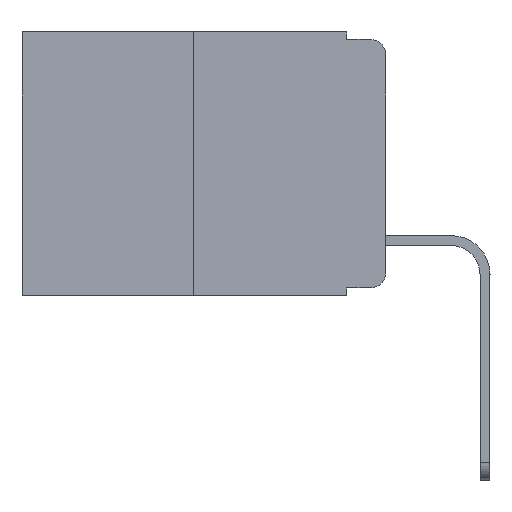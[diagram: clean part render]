
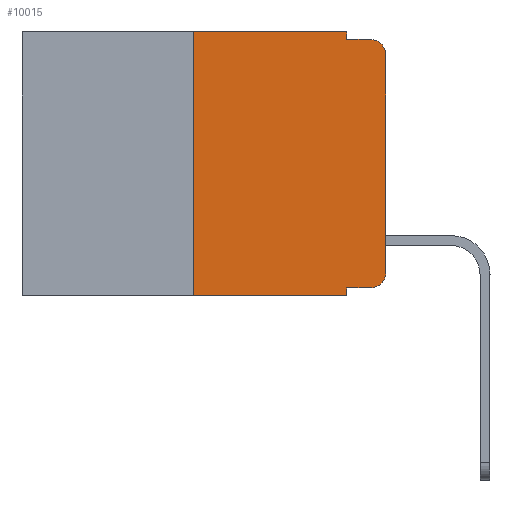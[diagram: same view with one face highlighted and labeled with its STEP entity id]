
A CAD part, left-side view. The second image highlights one B-rep face of the part: STEP entity #10015.
In plain terms, the highlighted planar face has unit normal (-1, 0, 0).
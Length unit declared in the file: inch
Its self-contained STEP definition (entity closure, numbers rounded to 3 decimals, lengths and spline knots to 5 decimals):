
#154 = CARTESIAN_POINT ( 'NONE',  ( 0., 0.051, -0.01 ) ) ;
#623 = ORIENTED_EDGE ( 'NONE', *, *, #19578, .F. ) ;
#699 = CARTESIAN_POINT ( 'NONE',  ( 0., 0.051, 0. ) ) ;
#938 = CARTESIAN_POINT ( 'NONE',  ( 0., 0.051, 0. ) ) ;
#1042 = DIRECTION ( 'NONE',  ( 0., 0., -1. ) ) ;
#1642 = EDGE_CURVE ( 'NONE', #15159, #14908, #9338, .T. ) ;
#1832 = VECTOR ( 'NONE', #19175, 39.37008 ) ;
#2206 = CARTESIAN_POINT ( 'NONE',  ( 0., 0.25, -0.343 ) ) ;
#2340 = ORIENTED_EDGE ( 'NONE', *, *, #16149, .F. ) ;
#3423 = VERTEX_POINT ( 'NONE', #938 ) ;
#4428 = LINE ( 'NONE', #9954, #6712 ) ;
#4862 = CARTESIAN_POINT ( 'NONE',  ( 0., 0., 0. ) ) ;
#5155 = AXIS2_PLACEMENT_3D ( 'NONE', #22812, #6828, #1042 ) ;
#5361 = VERTEX_POINT ( 'NONE', #21335 ) ;
#5397 = DIRECTION ( 'NONE',  ( -1., 0., 0. ) ) ;
#5840 = DIRECTION ( 'NONE',  ( 0., -1., 0. ) ) ;
#5917 = CARTESIAN_POINT ( 'NONE',  ( 0., 0.473, -0.343 ) ) ;
#6068 = DIRECTION ( 'NONE',  ( 0., -1., 0. ) ) ;
#6484 = ORIENTED_EDGE ( 'NONE', *, *, #8996, .T. ) ;
#6598 = DIRECTION ( 'NONE',  ( 0., 0., 1. ) ) ;
#6642 = VERTEX_POINT ( 'NONE', #8885 ) ;
#6712 = VECTOR ( 'NONE', #15363, 39.37008 ) ;
#6759 = DIRECTION ( 'NONE',  ( 0., 0., -1. ) ) ;
#6828 = DIRECTION ( 'NONE',  ( 1., 0., 0. ) ) ;
#6889 = ORIENTED_EDGE ( 'NONE', *, *, #14676, .F. ) ;
#6908 = DIRECTION ( 'NONE',  ( 0., 0., 1. ) ) ;
#7528 = LINE ( 'NONE', #17370, #1832 ) ;
#8420 = EDGE_LOOP ( 'NONE', ( #10664, #22888, #6889, #17474, #623, #2340, #9240, #12591, #6484, #17768 ) ) ;
#8558 = DIRECTION ( 'NONE',  ( 0., -1., 0. ) ) ;
#8692 = EDGE_CURVE ( 'NONE', #20101, #14908, #9041, .T. ) ;
#8847 = AXIS2_PLACEMENT_3D ( 'NONE', #14460, #5397, #14536 ) ;
#8885 = CARTESIAN_POINT ( 'NONE',  ( 0., 0., -0.313 ) ) ;
#8996 = EDGE_CURVE ( 'NONE', #20101, #19986, #18579, .T. ) ;
#9041 = LINE ( 'NONE', #699, #17463 ) ;
#9240 = ORIENTED_EDGE ( 'NONE', *, *, #1642, .T. ) ;
#9338 = LINE ( 'NONE', #5917, #22549 ) ;
#9572 = LINE ( 'NONE', #12081, #19370 ) ;
#9954 = CARTESIAN_POINT ( 'NONE',  ( 0., 0.051, 0. ) ) ;
#10015 = ADVANCED_FACE ( 'NONE', ( #12561 ), #15786, .F. ) ;
#10626 = CIRCLE ( 'NONE', #14514, 0.02 ) ;
#10664 = ORIENTED_EDGE ( 'NONE', *, *, #19601, .T. ) ;
#11359 = VERTEX_POINT ( 'NONE', #17925 ) ;
#11551 = CARTESIAN_POINT ( 'NONE',  ( 0., 0.02, -0.333 ) ) ;
#12081 = CARTESIAN_POINT ( 'NONE',  ( 0., 0.051, -0.01 ) ) ;
#12561 = FACE_OUTER_BOUND ( 'NONE', #8420, .T. ) ;
#12591 = ORIENTED_EDGE ( 'NONE', *, *, #8692, .F. ) ;
#13172 = DIRECTION ( 'NONE',  ( 0., 0., -1. ) ) ;
#14460 = CARTESIAN_POINT ( 'NONE',  ( 0., 0.02, -0.03 ) ) ;
#14514 = AXIS2_PLACEMENT_3D ( 'NONE', #17535, #22961, #6759 ) ;
#14536 = DIRECTION ( 'NONE',  ( 0., 0., -1. ) ) ;
#14676 = EDGE_CURVE ( 'NONE', #20392, #11359, #9572, .T. ) ;
#14908 = VERTEX_POINT ( 'NONE', #23185 ) ;
#15159 = VERTEX_POINT ( 'NONE', #2206 ) ;
#15363 = DIRECTION ( 'NONE',  ( 0., 0., -1. ) ) ;
#15467 = CARTESIAN_POINT ( 'NONE',  ( 0., 0.051, -0.333 ) ) ;
#15786 = PLANE ( 'NONE',  #5155 ) ;
#16149 = EDGE_CURVE ( 'NONE', #15159, #19144, #21340, .T. ) ;
#17370 = CARTESIAN_POINT ( 'NONE',  ( 0., 0.473, 0. ) ) ;
#17447 = VECTOR ( 'NONE', #5840, 39.37008 ) ;
#17463 = VECTOR ( 'NONE', #13172, 39.37008 ) ;
#17474 = ORIENTED_EDGE ( 'NONE', *, *, #18771, .F. ) ;
#17535 = CARTESIAN_POINT ( 'NONE',  ( 0., 0.02, -0.313 ) ) ;
#17768 = ORIENTED_EDGE ( 'NONE', *, *, #19514, .T. ) ;
#17925 = CARTESIAN_POINT ( 'NONE',  ( 0., 0.02, -0.01 ) ) ;
#18579 = LINE ( 'NONE', #20286, #17447 ) ;
#18771 = EDGE_CURVE ( 'NONE', #3423, #20392, #4428, .T. ) ;
#19144 = VERTEX_POINT ( 'NONE', #21785 ) ;
#19175 = DIRECTION ( 'NONE',  ( 0., -1., 0. ) ) ;
#19370 = VECTOR ( 'NONE', #8558, 39.37008 ) ;
#19485 = CIRCLE ( 'NONE', #8847, 0.02 ) ;
#19514 = EDGE_CURVE ( 'NONE', #19986, #6642, #10626, .T. ) ;
#19578 = EDGE_CURVE ( 'NONE', #19144, #3423, #7528, .T. ) ;
#19601 = EDGE_CURVE ( 'NONE', #6642, #5361, #19869, .T. ) ;
#19869 = LINE ( 'NONE', #4862, #21877 ) ;
#19986 = VERTEX_POINT ( 'NONE', #11551 ) ;
#20101 = VERTEX_POINT ( 'NONE', #15467 ) ;
#20286 = CARTESIAN_POINT ( 'NONE',  ( 0., 0.051, -0.333 ) ) ;
#20392 = VERTEX_POINT ( 'NONE', #154 ) ;
#20486 = VECTOR ( 'NONE', #6598, 39.37008 ) ;
#21335 = CARTESIAN_POINT ( 'NONE',  ( 0., 0., -0.03 ) ) ;
#21340 = LINE ( 'NONE', #22564, #20486 ) ;
#21785 = CARTESIAN_POINT ( 'NONE',  ( 0., 0.25, 0. ) ) ;
#21877 = VECTOR ( 'NONE', #6908, 39.37008 ) ;
#22549 = VECTOR ( 'NONE', #6068, 39.37008 ) ;
#22564 = CARTESIAN_POINT ( 'NONE',  ( 0., 0.25, 0. ) ) ;
#22812 = CARTESIAN_POINT ( 'NONE',  ( 0., 0.473, 0. ) ) ;
#22850 = EDGE_CURVE ( 'NONE', #5361, #11359, #19485, .T. ) ;
#22888 = ORIENTED_EDGE ( 'NONE', *, *, #22850, .T. ) ;
#22961 = DIRECTION ( 'NONE',  ( -1., 0., 0. ) ) ;
#23185 = CARTESIAN_POINT ( 'NONE',  ( 0., 0.051, -0.343 ) ) ;
